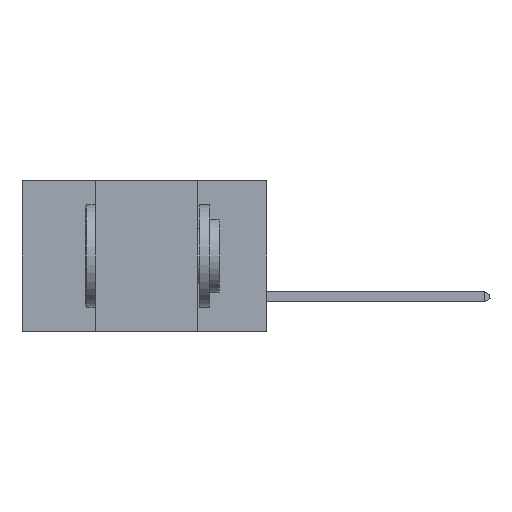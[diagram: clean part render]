
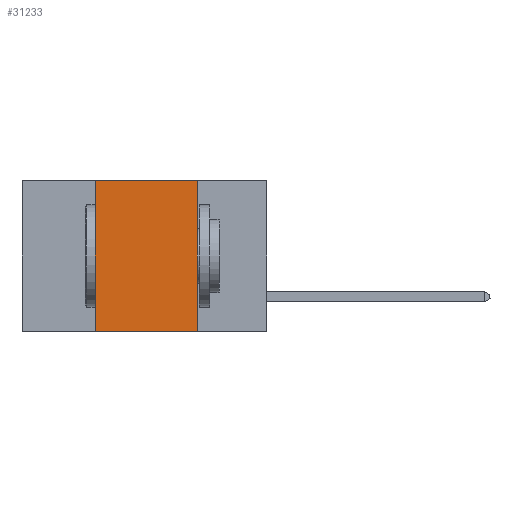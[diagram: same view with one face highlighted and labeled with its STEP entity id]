
A CAD part, left-side view. The second image highlights one B-rep face of the part: STEP entity #31233.
In plain terms, the highlighted planar face has unit normal (-1, 0, 0).
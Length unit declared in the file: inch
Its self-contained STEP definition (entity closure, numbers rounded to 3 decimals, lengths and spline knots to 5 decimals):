
#501 = CARTESIAN_POINT ( 'NONE',  ( 0., 0.17, 0. ) ) ;
#682 = DIRECTION ( 'NONE',  ( 0., 0., -1. ) ) ;
#2194 = ORIENTED_EDGE ( 'NONE', *, *, #42420, .F. ) ;
#4524 = VECTOR ( 'NONE', #16914, 39.37008 ) ;
#5308 = CARTESIAN_POINT ( 'NONE',  ( 0., 0.6, -0.37 ) ) ;
#9996 = CARTESIAN_POINT ( 'NONE',  ( 0., 0.6, 0. ) ) ;
#10620 = CARTESIAN_POINT ( 'NONE',  ( 0., 0.17, -0.37 ) ) ;
#11376 = FACE_OUTER_BOUND ( 'NONE', #46043, .T. ) ;
#13971 = DIRECTION ( 'NONE',  ( 0., 0., -1. ) ) ;
#15713 = EDGE_CURVE ( 'NONE', #48982, #23854, #40540, .T. ) ;
#16914 = DIRECTION ( 'NONE',  ( 0., 0., 1. ) ) ;
#20579 = CARTESIAN_POINT ( 'NONE',  ( 0., 0.42, 0. ) ) ;
#21609 = CARTESIAN_POINT ( 'NONE',  ( 0., 0.17, 0. ) ) ;
#21625 = DIRECTION ( 'NONE',  ( 1., 0., 0. ) ) ;
#21750 = CARTESIAN_POINT ( 'NONE',  ( 0., 0.42, 0. ) ) ;
#23671 = ORIENTED_EDGE ( 'NONE', *, *, #40362, .F. ) ;
#23854 = VERTEX_POINT ( 'NONE', #10620 ) ;
#24903 = VERTEX_POINT ( 'NONE', #21750 ) ;
#24938 = PLANE ( 'NONE',  #45411 ) ;
#25368 = DIRECTION ( 'NONE',  ( 0., -1., 0. ) ) ;
#26502 = LINE ( 'NONE', #501, #45454 ) ;
#28134 = VECTOR ( 'NONE', #25368, 39.37008 ) ;
#29487 = CARTESIAN_POINT ( 'NONE',  ( 0., 0.6, 0. ) ) ;
#30652 = VERTEX_POINT ( 'NONE', #21609 ) ;
#31233 = ADVANCED_FACE ( 'NONE', ( #11376 ), #24938, .F. ) ;
#31870 = DIRECTION ( 'NONE',  ( 0., -1., 0. ) ) ;
#36805 = EDGE_CURVE ( 'NONE', #24903, #30652, #38261, .T. ) ;
#38261 = LINE ( 'NONE', #29487, #28134 ) ;
#38454 = LINE ( 'NONE', #20579, #4524 ) ;
#39119 = ORIENTED_EDGE ( 'NONE', *, *, #36805, .F. ) ;
#40362 = EDGE_CURVE ( 'NONE', #48982, #24903, #38454, .T. ) ;
#40540 = LINE ( 'NONE', #5308, #45848 ) ;
#42420 = EDGE_CURVE ( 'NONE', #30652, #23854, #26502, .T. ) ;
#44316 = ORIENTED_EDGE ( 'NONE', *, *, #15713, .T. ) ;
#45411 = AXIS2_PLACEMENT_3D ( 'NONE', #9996, #21625, #13971 ) ;
#45428 = CARTESIAN_POINT ( 'NONE',  ( 0., 0.42, -0.37 ) ) ;
#45454 = VECTOR ( 'NONE', #682, 39.37008 ) ;
#45848 = VECTOR ( 'NONE', #31870, 39.37008 ) ;
#46043 = EDGE_LOOP ( 'NONE', ( #2194, #39119, #23671, #44316 ) ) ;
#48982 = VERTEX_POINT ( 'NONE', #45428 ) ;
